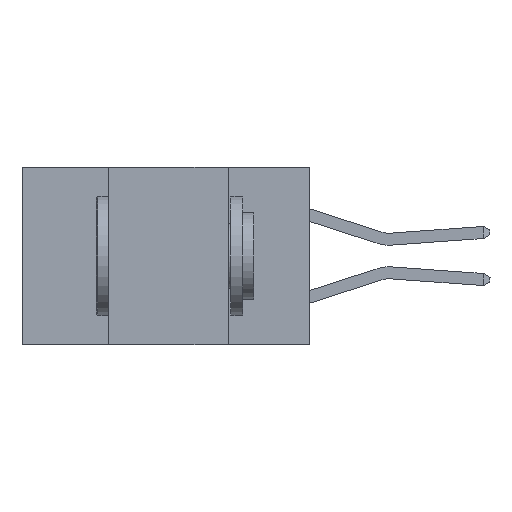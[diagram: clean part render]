
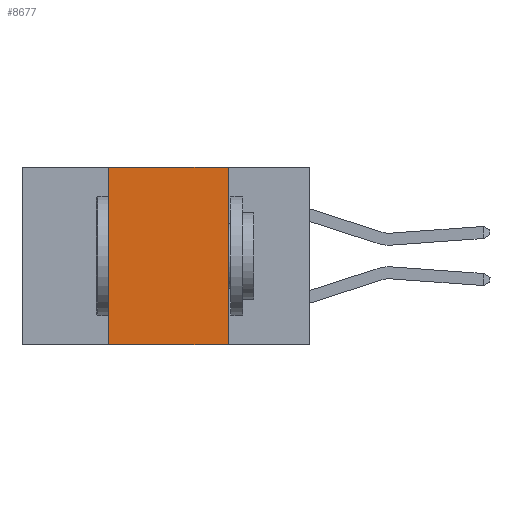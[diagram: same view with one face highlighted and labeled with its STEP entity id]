
A CAD part, left-side view. The second image highlights one B-rep face of the part: STEP entity #8677.
In plain terms, the highlighted planar face has unit normal (-1, 0, 0).
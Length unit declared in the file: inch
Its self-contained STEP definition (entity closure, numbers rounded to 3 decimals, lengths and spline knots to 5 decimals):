
#791 = EDGE_CURVE ( 'NONE', #18121, #11458, #3149, .T. ) ;
#2064 = VERTEX_POINT ( 'NONE', #3600 ) ;
#3149 = LINE ( 'NONE', #18438, #22667 ) ;
#3214 = ORIENTED_EDGE ( 'NONE', *, *, #16642, .F. ) ;
#3351 = EDGE_CURVE ( 'NONE', #18121, #2064, #8193, .T. ) ;
#3600 = CARTESIAN_POINT ( 'NONE',  ( 0., 0.42, 0. ) ) ;
#3884 = DIRECTION ( 'NONE',  ( 0., -1., 0. ) ) ;
#3945 = PLANE ( 'NONE',  #23081 ) ;
#3970 = VECTOR ( 'NONE', #17068, 39.37008 ) ;
#4048 = CARTESIAN_POINT ( 'NONE',  ( 0., 0.17, -0.37 ) ) ;
#4547 = FACE_OUTER_BOUND ( 'NONE', #6493, .T. ) ;
#6493 = EDGE_LOOP ( 'NONE', ( #3214, #12427, #16682, #11856 ) ) ;
#7649 = DIRECTION ( 'NONE',  ( 1., 0., 0. ) ) ;
#7716 = LINE ( 'NONE', #15269, #3970 ) ;
#8193 = LINE ( 'NONE', #17928, #21643 ) ;
#8480 = VECTOR ( 'NONE', #18715, 39.37008 ) ;
#8677 = ADVANCED_FACE ( 'NONE', ( #4547 ), #3945, .F. ) ;
#9670 = VERTEX_POINT ( 'NONE', #10074 ) ;
#10074 = CARTESIAN_POINT ( 'NONE',  ( 0., 0.17, 0. ) ) ;
#11458 = VERTEX_POINT ( 'NONE', #21073 ) ;
#11856 = ORIENTED_EDGE ( 'NONE', *, *, #791, .T. ) ;
#12427 = ORIENTED_EDGE ( 'NONE', *, *, #21875, .F. ) ;
#13956 = LINE ( 'NONE', #4048, #8480 ) ;
#15269 = CARTESIAN_POINT ( 'NONE',  ( 0., 0.6, 0. ) ) ;
#16642 = EDGE_CURVE ( 'NONE', #9670, #11458, #13956, .T. ) ;
#16682 = ORIENTED_EDGE ( 'NONE', *, *, #3351, .F. ) ;
#16702 = DIRECTION ( 'NONE',  ( 0., 0., 1. ) ) ;
#17027 = CARTESIAN_POINT ( 'NONE',  ( 0., 0.42, -0.37 ) ) ;
#17068 = DIRECTION ( 'NONE',  ( 0., -1., 0. ) ) ;
#17928 = CARTESIAN_POINT ( 'NONE',  ( 0., 0.42, -0.37 ) ) ;
#18121 = VERTEX_POINT ( 'NONE', #17027 ) ;
#18438 = CARTESIAN_POINT ( 'NONE',  ( 0., 0.6, -0.37 ) ) ;
#18617 = CARTESIAN_POINT ( 'NONE',  ( 0., 0.6, 0. ) ) ;
#18715 = DIRECTION ( 'NONE',  ( 0., 0., -1. ) ) ;
#20473 = DIRECTION ( 'NONE',  ( 0., 0., -1. ) ) ;
#21073 = CARTESIAN_POINT ( 'NONE',  ( 0., 0.17, -0.37 ) ) ;
#21643 = VECTOR ( 'NONE', #16702, 39.37008 ) ;
#21875 = EDGE_CURVE ( 'NONE', #2064, #9670, #7716, .T. ) ;
#22667 = VECTOR ( 'NONE', #3884, 39.37008 ) ;
#23081 = AXIS2_PLACEMENT_3D ( 'NONE', #18617, #7649, #20473 ) ;
